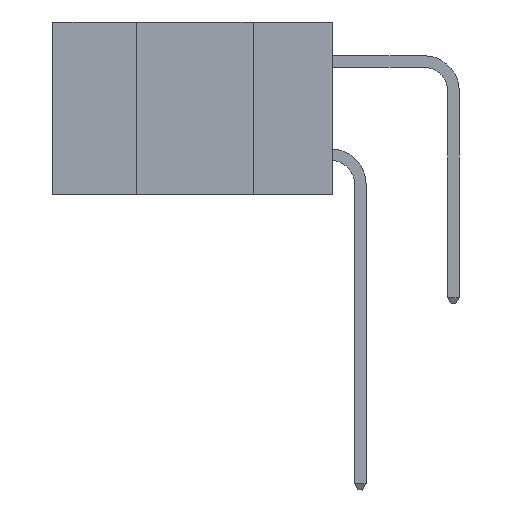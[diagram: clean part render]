
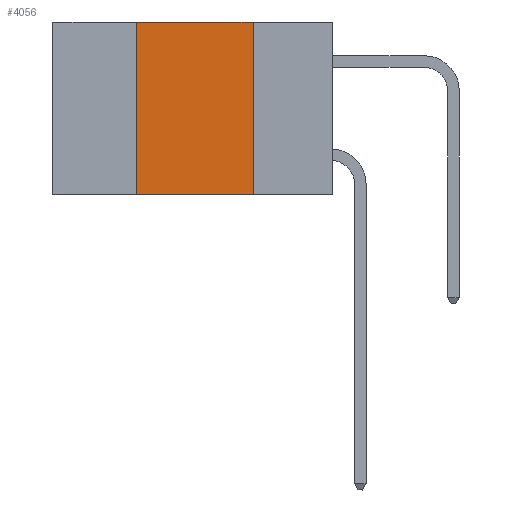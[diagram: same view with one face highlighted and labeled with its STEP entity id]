
A CAD part, left-side view. The second image highlights one B-rep face of the part: STEP entity #4056.
In plain terms, the highlighted planar face has unit normal (-1, 0, 0).
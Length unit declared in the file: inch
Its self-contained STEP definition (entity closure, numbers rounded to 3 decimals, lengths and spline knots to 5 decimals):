
#2 = CARTESIAN_POINT ( 'NONE',  ( 0., 0.17, 0. ) ) ;
#89 = DIRECTION ( 'NONE',  ( 0., 0., -1. ) ) ;
#108 = DIRECTION ( 'NONE',  ( 1., 0., 0. ) ) ;
#153 = ORIENTED_EDGE ( 'NONE', *, *, #4392, .T. ) ;
#157 = PLANE ( 'NONE',  #8859 ) ;
#381 = CARTESIAN_POINT ( 'NONE',  ( 0., 0.6, 0. ) ) ;
#628 = DIRECTION ( 'NONE',  ( 0., -1., 0. ) ) ;
#871 = LINE ( 'NONE', #7232, #1156 ) ;
#979 = EDGE_CURVE ( 'NONE', #1568, #1532, #10303, .T. ) ;
#1050 = DIRECTION ( 'NONE',  ( 0., 0., -1. ) ) ;
#1156 = VECTOR ( 'NONE', #89, 39.37008 ) ;
#1300 = DIRECTION ( 'NONE',  ( 0., 0., 1. ) ) ;
#1532 = VERTEX_POINT ( 'NONE', #11397 ) ;
#1568 = VERTEX_POINT ( 'NONE', #1713 ) ;
#1644 = EDGE_LOOP ( 'NONE', ( #5931, #10026, #2988, #153 ) ) ;
#1713 = CARTESIAN_POINT ( 'NONE',  ( 0., 0.42, -0.37 ) ) ;
#2187 = VERTEX_POINT ( 'NONE', #7205 ) ;
#2378 = LINE ( 'NONE', #4256, #3273 ) ;
#2988 = ORIENTED_EDGE ( 'NONE', *, *, #979, .F. ) ;
#3273 = VECTOR ( 'NONE', #628, 39.37008 ) ;
#3646 = FACE_OUTER_BOUND ( 'NONE', #1644, .T. ) ;
#3805 = DIRECTION ( 'NONE',  ( 0., -1., 0. ) ) ;
#4056 = ADVANCED_FACE ( 'NONE', ( #3646 ), #157, .F. ) ;
#4234 = EDGE_CURVE ( 'NONE', #1532, #10048, #9981, .T. ) ;
#4256 = CARTESIAN_POINT ( 'NONE',  ( 0., 0.6, -0.37 ) ) ;
#4392 = EDGE_CURVE ( 'NONE', #1568, #2187, #2378, .T. ) ;
#4494 = EDGE_CURVE ( 'NONE', #10048, #2187, #871, .T. ) ;
#5756 = VECTOR ( 'NONE', #3805, 39.37008 ) ;
#5931 = ORIENTED_EDGE ( 'NONE', *, *, #4494, .F. ) ;
#7205 = CARTESIAN_POINT ( 'NONE',  ( 0., 0.17, -0.37 ) ) ;
#7232 = CARTESIAN_POINT ( 'NONE',  ( 0., 0.17, -0.37 ) ) ;
#7888 = CARTESIAN_POINT ( 'NONE',  ( 0., 0.6, 0. ) ) ;
#8859 = AXIS2_PLACEMENT_3D ( 'NONE', #7888, #108, #1050 ) ;
#9251 = CARTESIAN_POINT ( 'NONE',  ( 0., 0.42, -0.37 ) ) ;
#9981 = LINE ( 'NONE', #381, #5756 ) ;
#10026 = ORIENTED_EDGE ( 'NONE', *, *, #4234, .F. ) ;
#10048 = VERTEX_POINT ( 'NONE', #2 ) ;
#10303 = LINE ( 'NONE', #9251, #10826 ) ;
#10826 = VECTOR ( 'NONE', #1300, 39.37008 ) ;
#11397 = CARTESIAN_POINT ( 'NONE',  ( 0., 0.42, 0. ) ) ;
